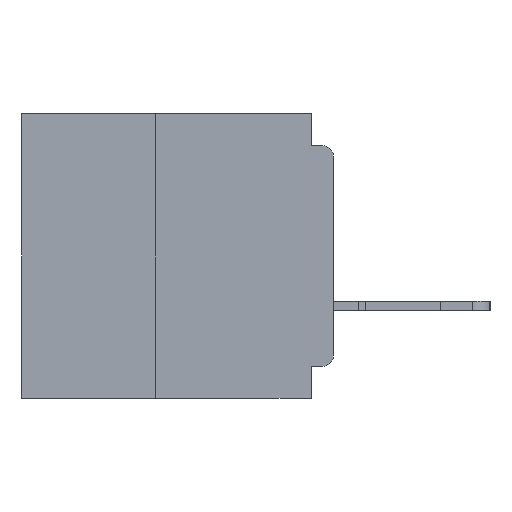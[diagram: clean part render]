
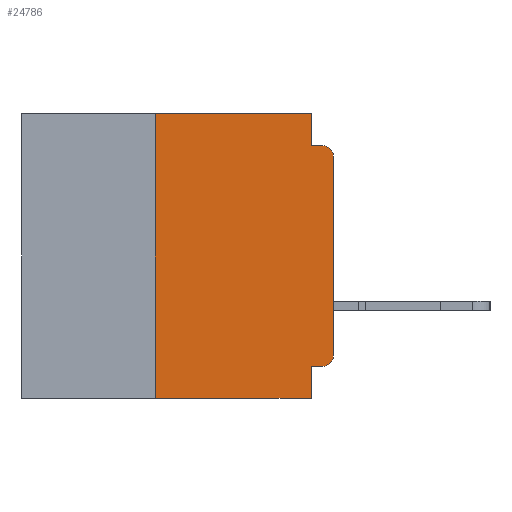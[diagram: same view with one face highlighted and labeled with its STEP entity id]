
A CAD part, left-side view. The second image highlights one B-rep face of the part: STEP entity #24786.
In plain terms, the highlighted planar face has unit normal (-1, 0, 0).
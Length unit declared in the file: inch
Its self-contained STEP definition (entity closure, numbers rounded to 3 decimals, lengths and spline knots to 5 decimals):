
#529 = ORIENTED_EDGE ( 'NONE', *, *, #24430, .F. ) ;
#799 = CARTESIAN_POINT ( 'NONE',  ( 0., 0.031, -0.4 ) ) ;
#2614 = VECTOR ( 'NONE', #21014, 39.37008 ) ;
#5290 = PLANE ( 'NONE',  #43978 ) ;
#6577 = VERTEX_POINT ( 'NONE', #33645 ) ;
#7020 = VERTEX_POINT ( 'NONE', #42327 ) ;
#7666 = VECTOR ( 'NONE', #62417, 39.37008 ) ;
#8492 = AXIS2_PLACEMENT_3D ( 'NONE', #19194, #53321, #24136 ) ;
#9339 = EDGE_CURVE ( 'NONE', #62664, #6577, #38315, .T. ) ;
#10013 = EDGE_CURVE ( 'NONE', #35895, #46825, #60206, .T. ) ;
#10224 = DIRECTION ( 'NONE',  ( 1., 0., 0. ) ) ;
#11054 = CARTESIAN_POINT ( 'NONE',  ( 0., 0.031, 0. ) ) ;
#11823 = ORIENTED_EDGE ( 'NONE', *, *, #50131, .T. ) ;
#12442 = LINE ( 'NONE', #29200, #49852 ) ;
#14727 = CARTESIAN_POINT ( 'NONE',  ( 0., 0.015, -0.06 ) ) ;
#16548 = EDGE_CURVE ( 'NONE', #33227, #62664, #23078, .T. ) ;
#17079 = CARTESIAN_POINT ( 'NONE',  ( 0., 0., -0.355 ) ) ;
#17351 = DIRECTION ( 'NONE',  ( 0., -1., 0. ) ) ;
#18527 = LINE ( 'NONE', #11054, #52865 ) ;
#18664 = CARTESIAN_POINT ( 'NONE',  ( 0., 0.437, -0.4 ) ) ;
#19153 = ORIENTED_EDGE ( 'NONE', *, *, #48885, .F. ) ;
#19194 = CARTESIAN_POINT ( 'NONE',  ( 0., 0.015, -0.34 ) ) ;
#19640 = DIRECTION ( 'NONE',  ( 0., 0., -1. ) ) ;
#19688 = DIRECTION ( 'NONE',  ( 0., -1., 0. ) ) ;
#20800 = LINE ( 'NONE', #17079, #56581 ) ;
#20870 = DIRECTION ( 'NONE',  ( 0., 0., -1. ) ) ;
#21014 = DIRECTION ( 'NONE',  ( 0., 0., -1. ) ) ;
#23078 = CIRCLE ( 'NONE', #8492, 0.015 ) ;
#23828 = VECTOR ( 'NONE', #50077, 39.37008 ) ;
#24136 = DIRECTION ( 'NONE',  ( 0., 0., -1. ) ) ;
#24411 = CARTESIAN_POINT ( 'NONE',  ( 0., 0., -0.045 ) ) ;
#24430 = EDGE_CURVE ( 'NONE', #33227, #42191, #20800, .T. ) ;
#24786 = ADVANCED_FACE ( 'NONE', ( #35260 ), #5290, .F. ) ;
#25572 = EDGE_CURVE ( 'NONE', #42191, #47498, #54546, .T. ) ;
#26681 = ORIENTED_EDGE ( 'NONE', *, *, #25572, .F. ) ;
#27583 = VERTEX_POINT ( 'NONE', #60133 ) ;
#29200 = CARTESIAN_POINT ( 'NONE',  ( 0., 0.25, -0.4 ) ) ;
#29635 = CARTESIAN_POINT ( 'NONE',  ( 0., 0.437, 0. ) ) ;
#30574 = ORIENTED_EDGE ( 'NONE', *, *, #10013, .F. ) ;
#30668 = CARTESIAN_POINT ( 'NONE',  ( 0., 0., 0. ) ) ;
#30833 = CARTESIAN_POINT ( 'NONE',  ( 0., 0.031, -0.4 ) ) ;
#31953 = ORIENTED_EDGE ( 'NONE', *, *, #57075, .F. ) ;
#33227 = VERTEX_POINT ( 'NONE', #44406 ) ;
#33645 = CARTESIAN_POINT ( 'NONE',  ( 0., 0., -0.06 ) ) ;
#34061 = DIRECTION ( 'NONE',  ( 0., 0., 1. ) ) ;
#34230 = VERTEX_POINT ( 'NONE', #58277 ) ;
#34367 = VECTOR ( 'NONE', #17351, 39.37008 ) ;
#35260 = FACE_OUTER_BOUND ( 'NONE', #56592, .T. ) ;
#35852 = LINE ( 'NONE', #24411, #45716 ) ;
#35895 = VERTEX_POINT ( 'NONE', #57248 ) ;
#37752 = CIRCLE ( 'NONE', #44099, 0.015 ) ;
#38315 = LINE ( 'NONE', #30668, #23828 ) ;
#39262 = EDGE_CURVE ( 'NONE', #27583, #47498, #59461, .T. ) ;
#39797 = CARTESIAN_POINT ( 'NONE',  ( 0., 0.031, 0. ) ) ;
#41974 = ORIENTED_EDGE ( 'NONE', *, *, #39262, .T. ) ;
#42191 = VERTEX_POINT ( 'NONE', #43199 ) ;
#42327 = CARTESIAN_POINT ( 'NONE',  ( 0., 0.031, -0.045 ) ) ;
#42513 = CARTESIAN_POINT ( 'NONE',  ( 0., 0., -0.34 ) ) ;
#43199 = CARTESIAN_POINT ( 'NONE',  ( 0., 0.031, -0.355 ) ) ;
#43978 = AXIS2_PLACEMENT_3D ( 'NONE', #29635, #10224, #44297 ) ;
#44099 = AXIS2_PLACEMENT_3D ( 'NONE', #14727, #48870, #19640 ) ;
#44297 = DIRECTION ( 'NONE',  ( 0., 0., -1. ) ) ;
#44406 = CARTESIAN_POINT ( 'NONE',  ( 0., 0.015, -0.355 ) ) ;
#45171 = ORIENTED_EDGE ( 'NONE', *, *, #9339, .T. ) ;
#45716 = VECTOR ( 'NONE', #19688, 39.37008 ) ;
#46825 = VERTEX_POINT ( 'NONE', #39797 ) ;
#47498 = VERTEX_POINT ( 'NONE', #799 ) ;
#47762 = ORIENTED_EDGE ( 'NONE', *, *, #16548, .T. ) ;
#48870 = DIRECTION ( 'NONE',  ( -1., 0., 0. ) ) ;
#48885 = EDGE_CURVE ( 'NONE', #27583, #35895, #12442, .T. ) ;
#49852 = VECTOR ( 'NONE', #34061, 39.37008 ) ;
#50077 = DIRECTION ( 'NONE',  ( 0., 0., 1. ) ) ;
#50131 = EDGE_CURVE ( 'NONE', #6577, #34230, #37752, .T. ) ;
#51138 = EDGE_CURVE ( 'NONE', #46825, #7020, #18527, .T. ) ;
#51485 = CARTESIAN_POINT ( 'NONE',  ( 0., 0.437, 0. ) ) ;
#52865 = VECTOR ( 'NONE', #20870, 39.37008 ) ;
#53321 = DIRECTION ( 'NONE',  ( -1., 0., 0. ) ) ;
#54546 = LINE ( 'NONE', #30833, #2614 ) ;
#56059 = DIRECTION ( 'NONE',  ( 0., 1., 0. ) ) ;
#56581 = VECTOR ( 'NONE', #56059, 39.37008 ) ;
#56592 = EDGE_LOOP ( 'NONE', ( #45171, #11823, #31953, #60521, #30574, #19153, #41974, #26681, #529, #47762 ) ) ;
#57075 = EDGE_CURVE ( 'NONE', #7020, #34230, #35852, .T. ) ;
#57248 = CARTESIAN_POINT ( 'NONE',  ( 0., 0.25, 0. ) ) ;
#58277 = CARTESIAN_POINT ( 'NONE',  ( 0., 0.015, -0.045 ) ) ;
#59461 = LINE ( 'NONE', #18664, #7666 ) ;
#60133 = CARTESIAN_POINT ( 'NONE',  ( 0., 0.25, -0.4 ) ) ;
#60206 = LINE ( 'NONE', #51485, #34367 ) ;
#60521 = ORIENTED_EDGE ( 'NONE', *, *, #51138, .F. ) ;
#62417 = DIRECTION ( 'NONE',  ( 0., -1., 0. ) ) ;
#62664 = VERTEX_POINT ( 'NONE', #42513 ) ;
